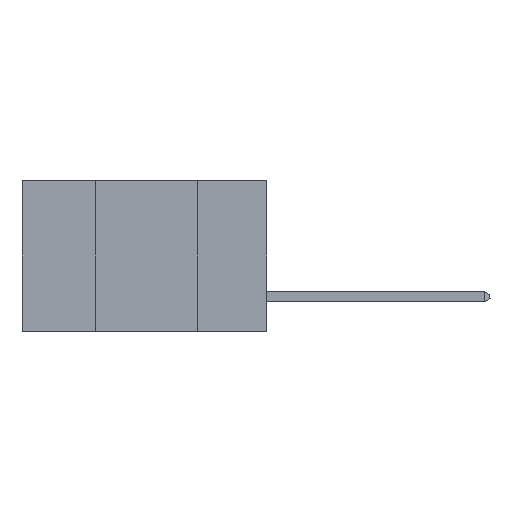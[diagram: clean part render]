
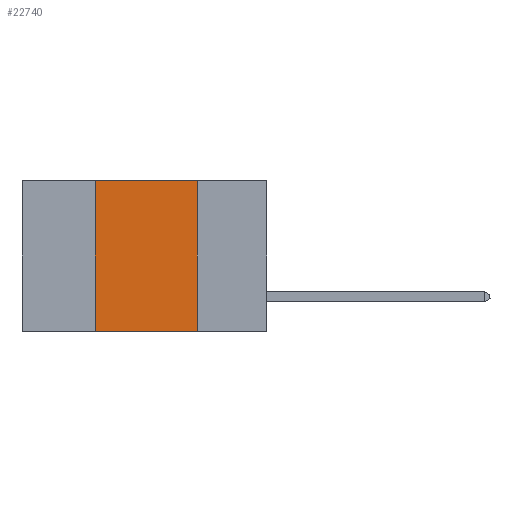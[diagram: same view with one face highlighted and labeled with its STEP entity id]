
A CAD part, left-side view. The second image highlights one B-rep face of the part: STEP entity #22740.
In plain terms, the highlighted planar face has unit normal (-1, 0, 0).
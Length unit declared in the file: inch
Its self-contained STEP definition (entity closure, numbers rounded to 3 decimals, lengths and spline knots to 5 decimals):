
#1677 = DIRECTION ( 'NONE',  ( 0., 0., -1. ) ) ;
#1743 = ORIENTED_EDGE ( 'NONE', *, *, #12863, .F. ) ;
#2608 = VERTEX_POINT ( 'NONE', #23071 ) ;
#4632 = EDGE_LOOP ( 'NONE', ( #9225, #1743, #18864, #17483 ) ) ;
#5031 = DIRECTION ( 'NONE',  ( 0., 0., -1. ) ) ;
#5151 = EDGE_CURVE ( 'NONE', #25534, #2608, #14821, .T. ) ;
#5514 = DIRECTION ( 'NONE',  ( 0., -1., 0. ) ) ;
#6219 = CARTESIAN_POINT ( 'NONE',  ( 0., 0.17, 0. ) ) ;
#7725 = LINE ( 'NONE', #18151, #8079 ) ;
#8079 = VECTOR ( 'NONE', #5514, 39.37008 ) ;
#8995 = CARTESIAN_POINT ( 'NONE',  ( 0., 0.17, -0.37 ) ) ;
#9037 = VERTEX_POINT ( 'NONE', #22594 ) ;
#9225 = ORIENTED_EDGE ( 'NONE', *, *, #20579, .F. ) ;
#9291 = DIRECTION ( 'NONE',  ( 1., 0., 0. ) ) ;
#9848 = VECTOR ( 'NONE', #18974, 39.37008 ) ;
#9903 = CARTESIAN_POINT ( 'NONE',  ( 0., 0.6, -0.37 ) ) ;
#11996 = LINE ( 'NONE', #6219, #23696 ) ;
#12863 = EDGE_CURVE ( 'NONE', #2608, #9037, #7725, .T. ) ;
#14821 = LINE ( 'NONE', #27220, #22593 ) ;
#15277 = CARTESIAN_POINT ( 'NONE',  ( 0., 0.42, -0.37 ) ) ;
#15746 = DIRECTION ( 'NONE',  ( 0., 0., 1. ) ) ;
#15828 = EDGE_CURVE ( 'NONE', #25534, #18160, #25035, .T. ) ;
#16269 = PLANE ( 'NONE',  #26940 ) ;
#17483 = ORIENTED_EDGE ( 'NONE', *, *, #15828, .T. ) ;
#18151 = CARTESIAN_POINT ( 'NONE',  ( 0., 0.6, 0. ) ) ;
#18160 = VERTEX_POINT ( 'NONE', #8995 ) ;
#18539 = CARTESIAN_POINT ( 'NONE',  ( 0., 0.6, 0. ) ) ;
#18864 = ORIENTED_EDGE ( 'NONE', *, *, #5151, .F. ) ;
#18974 = DIRECTION ( 'NONE',  ( 0., -1., 0. ) ) ;
#20579 = EDGE_CURVE ( 'NONE', #9037, #18160, #11996, .T. ) ;
#22593 = VECTOR ( 'NONE', #15746, 39.37008 ) ;
#22594 = CARTESIAN_POINT ( 'NONE',  ( 0., 0.17, 0. ) ) ;
#22740 = ADVANCED_FACE ( 'NONE', ( #23500 ), #16269, .F. ) ;
#23071 = CARTESIAN_POINT ( 'NONE',  ( 0., 0.42, 0. ) ) ;
#23500 = FACE_OUTER_BOUND ( 'NONE', #4632, .T. ) ;
#23696 = VECTOR ( 'NONE', #1677, 39.37008 ) ;
#25035 = LINE ( 'NONE', #9903, #9848 ) ;
#25534 = VERTEX_POINT ( 'NONE', #15277 ) ;
#26940 = AXIS2_PLACEMENT_3D ( 'NONE', #18539, #9291, #5031 ) ;
#27220 = CARTESIAN_POINT ( 'NONE',  ( 0., 0.42, 0. ) ) ;
